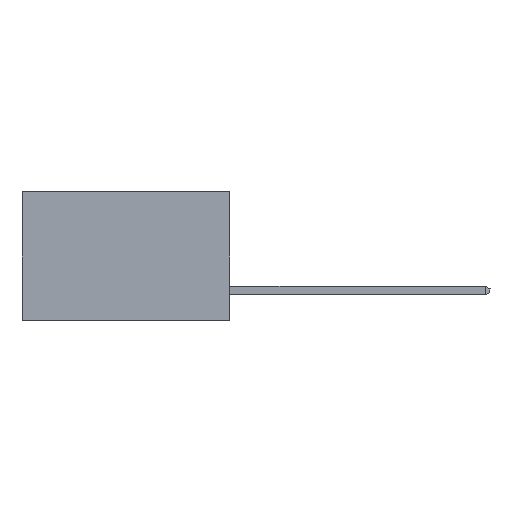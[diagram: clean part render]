
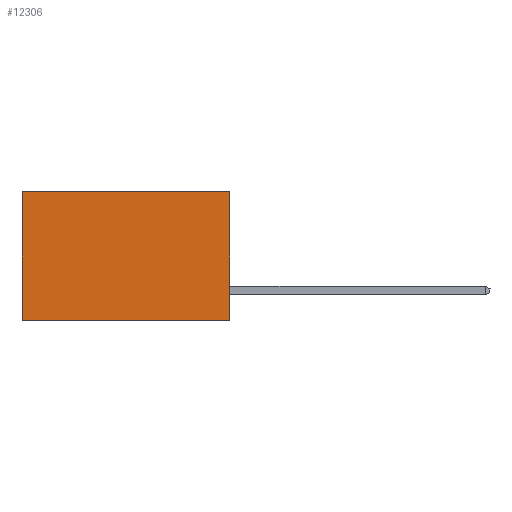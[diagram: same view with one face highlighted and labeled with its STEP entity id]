
A CAD part, left-side view. The second image highlights one B-rep face of the part: STEP entity #12306.
In plain terms, the highlighted planar face has unit normal (-1, 0, 0).
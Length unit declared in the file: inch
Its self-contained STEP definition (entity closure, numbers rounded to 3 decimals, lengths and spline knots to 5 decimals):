
#508 = CARTESIAN_POINT ( 'NONE',  ( 0.2615, 0., -0.37 ) ) ;
#664 = VECTOR ( 'NONE', #16940, 39.37008 ) ;
#713 = DIRECTION ( 'NONE',  ( 0., 0., -1. ) ) ;
#860 = DIRECTION ( 'NONE',  ( 0., 1., 0. ) ) ;
#887 = ORIENTED_EDGE ( 'NONE', *, *, #12042, .F. ) ;
#2001 = VECTOR ( 'NONE', #5442, 39.37008 ) ;
#2169 = CARTESIAN_POINT ( 'NONE',  ( 0.2615, 0., 0. ) ) ;
#2260 = LINE ( 'NONE', #5736, #664 ) ;
#2268 = AXIS2_PLACEMENT_3D ( 'NONE', #508, #20163, #713 ) ;
#2880 = VERTEX_POINT ( 'NONE', #14904 ) ;
#2912 = VERTEX_POINT ( 'NONE', #7284 ) ;
#3694 = EDGE_CURVE ( 'NONE', #6340, #17098, #2260, .T. ) ;
#4233 = VECTOR ( 'NONE', #19750, 39.37008 ) ;
#4617 = VECTOR ( 'NONE', #860, 39.37008 ) ;
#5442 = DIRECTION ( 'NONE',  ( 0., 0., -1. ) ) ;
#5736 = CARTESIAN_POINT ( 'NONE',  ( 0.2615, 0., -0.37 ) ) ;
#6056 = ORIENTED_EDGE ( 'NONE', *, *, #3694, .F. ) ;
#6340 = VERTEX_POINT ( 'NONE', #2169 ) ;
#6852 = LINE ( 'NONE', #13299, #4233 ) ;
#7152 = ORIENTED_EDGE ( 'NONE', *, *, #18875, .T. ) ;
#7161 = FACE_OUTER_BOUND ( 'NONE', #11290, .T. ) ;
#7284 = CARTESIAN_POINT ( 'NONE',  ( 0.2615, 0.6, -0.37 ) ) ;
#7321 = LINE ( 'NONE', #18514, #2001 ) ;
#7711 = ORIENTED_EDGE ( 'NONE', *, *, #12288, .T. ) ;
#8202 = CARTESIAN_POINT ( 'NONE',  ( 0.2615, 0., -0.37 ) ) ;
#10236 = PLANE ( 'NONE',  #2268 ) ;
#11290 = EDGE_LOOP ( 'NONE', ( #7152, #887, #6056, #7711 ) ) ;
#12042 = EDGE_CURVE ( 'NONE', #17098, #2912, #20210, .T. ) ;
#12288 = EDGE_CURVE ( 'NONE', #6340, #2880, #6852, .T. ) ;
#12306 = ADVANCED_FACE ( 'NONE', ( #7161 ), #10236, .F. ) ;
#13299 = CARTESIAN_POINT ( 'NONE',  ( 0.2615, 0., 0. ) ) ;
#14904 = CARTESIAN_POINT ( 'NONE',  ( 0.2615, 0.6, 0. ) ) ;
#16940 = DIRECTION ( 'NONE',  ( 0., 0., -1. ) ) ;
#17098 = VERTEX_POINT ( 'NONE', #8202 ) ;
#18514 = CARTESIAN_POINT ( 'NONE',  ( 0.2615, 0.6, -0.37 ) ) ;
#18714 = CARTESIAN_POINT ( 'NONE',  ( 0.2615, 0., -0.37 ) ) ;
#18875 = EDGE_CURVE ( 'NONE', #2880, #2912, #7321, .T. ) ;
#19750 = DIRECTION ( 'NONE',  ( 0., 1., 0. ) ) ;
#20163 = DIRECTION ( 'NONE',  ( 1., 0., 0. ) ) ;
#20210 = LINE ( 'NONE', #18714, #4617 ) ;
